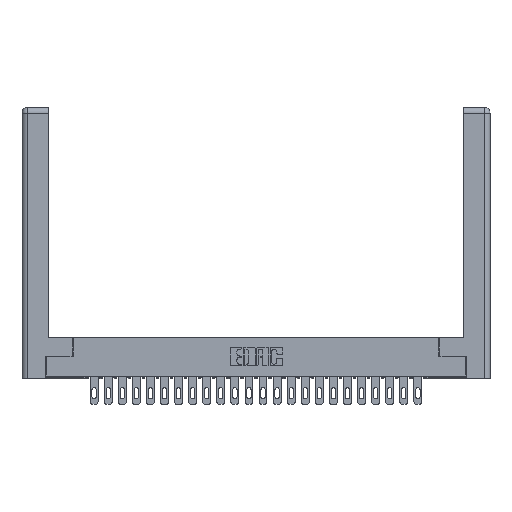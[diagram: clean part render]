
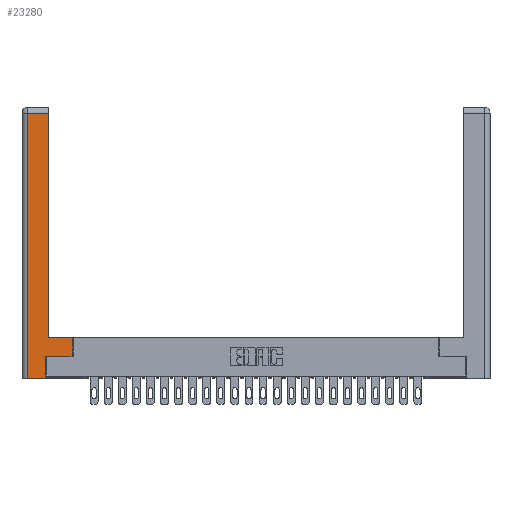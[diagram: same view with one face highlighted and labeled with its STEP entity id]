
A CAD part, top view. The second image highlights one B-rep face of the part: STEP entity #23280.
In plain terms, the highlighted planar face has unit normal (0, 0, 1).
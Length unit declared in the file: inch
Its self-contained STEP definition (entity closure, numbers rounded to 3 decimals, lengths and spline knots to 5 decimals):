
#617 = DIRECTION ( 'NONE',  ( -1., 0., 0. ) ) ;
#824 = EDGE_LOOP ( 'NONE', ( #2132, #4678, #20342, #11618, #15041, #20733, #7342, #21084 ) ) ;
#1016 = DIRECTION ( 'NONE',  ( 1., 0., 0. ) ) ;
#1511 = VECTOR ( 'NONE', #1597, 39.37008 ) ;
#1597 = DIRECTION ( 'NONE',  ( 1., 0., 0. ) ) ;
#1725 = CARTESIAN_POINT ( 'NONE',  ( 0.565, 0.245, 0. ) ) ;
#2132 = ORIENTED_EDGE ( 'NONE', *, *, #16651, .T. ) ;
#2185 = LINE ( 'NONE', #14573, #8095 ) ;
#2414 = CARTESIAN_POINT ( 'NONE',  ( 0.295, 2.94, 0. ) ) ;
#3027 = CARTESIAN_POINT ( 'NONE',  ( 0.565, 0.45, 0. ) ) ;
#3038 = DIRECTION ( 'NONE',  ( 0., 1., 0. ) ) ;
#3430 = EDGE_CURVE ( 'NONE', #23689, #16649, #26467, .T. ) ;
#3661 = CARTESIAN_POINT ( 'NONE',  ( 0.565, 0.45, 0. ) ) ;
#4438 = DIRECTION ( 'NONE',  ( -1., 0., 0. ) ) ;
#4440 = CARTESIAN_POINT ( 'NONE',  ( 0.0615, 2.94, 0. ) ) ;
#4678 = ORIENTED_EDGE ( 'NONE', *, *, #17542, .T. ) ;
#4909 = CARTESIAN_POINT ( 'NONE',  ( 0.295, 3., 0. ) ) ;
#5055 = DIRECTION ( 'NONE',  ( 0., 1., 0. ) ) ;
#5599 = DIRECTION ( 'NONE',  ( 0., 1., 0. ) ) ;
#5672 = LINE ( 'NONE', #19883, #8420 ) ;
#6234 = CARTESIAN_POINT ( 'NONE',  ( 0.265, 0.245, 0. ) ) ;
#7342 = ORIENTED_EDGE ( 'NONE', *, *, #8718, .T. ) ;
#8095 = VECTOR ( 'NONE', #8849, 39.37008 ) ;
#8358 = CARTESIAN_POINT ( 'NONE',  ( 0., 0., 0. ) ) ;
#8420 = VECTOR ( 'NONE', #3038, 39.37008 ) ;
#8718 = EDGE_CURVE ( 'NONE', #16969, #22147, #22733, .T. ) ;
#8766 = PLANE ( 'NONE',  #25941 ) ;
#8849 = DIRECTION ( 'NONE',  ( 0., -1., 0. ) ) ;
#10467 = EDGE_CURVE ( 'NONE', #22147, #15799, #21754, .T. ) ;
#11216 = LINE ( 'NONE', #4909, #23379 ) ;
#11480 = EDGE_CURVE ( 'NONE', #16649, #21962, #5672, .T. ) ;
#11585 = CARTESIAN_POINT ( 'NONE',  ( 0.295, 0.45, 0. ) ) ;
#11618 = ORIENTED_EDGE ( 'NONE', *, *, #3430, .T. ) ;
#11928 = LINE ( 'NONE', #12333, #1511 ) ;
#12333 = CARTESIAN_POINT ( 'NONE',  ( 0.565, 0.245, 0. ) ) ;
#12905 = EDGE_CURVE ( 'NONE', #21962, #16969, #11928, .T. ) ;
#13157 = CARTESIAN_POINT ( 'NONE',  ( 0.295, 0.45, 0. ) ) ;
#13964 = CARTESIAN_POINT ( 'NONE',  ( 0.265, 0., 0. ) ) ;
#14573 = CARTESIAN_POINT ( 'NONE',  ( 0.0615, 0., 0. ) ) ;
#15041 = ORIENTED_EDGE ( 'NONE', *, *, #11480, .T. ) ;
#15799 = VERTEX_POINT ( 'NONE', #11585 ) ;
#16649 = VERTEX_POINT ( 'NONE', #19810 ) ;
#16651 = EDGE_CURVE ( 'NONE', #15799, #22314, #11216, .T. ) ;
#16969 = VERTEX_POINT ( 'NONE', #1725 ) ;
#17184 = VECTOR ( 'NONE', #5599, 39.37008 ) ;
#17542 = EDGE_CURVE ( 'NONE', #22314, #25820, #23534, .T. ) ;
#17714 = VECTOR ( 'NONE', #617, 39.37008 ) ;
#18211 = VECTOR ( 'NONE', #1016, 39.37008 ) ;
#18789 = FACE_OUTER_BOUND ( 'NONE', #824, .T. ) ;
#19810 = CARTESIAN_POINT ( 'NONE',  ( 0.265, 0., 0. ) ) ;
#19883 = CARTESIAN_POINT ( 'NONE',  ( 0.265, 0.245, 0. ) ) ;
#20342 = ORIENTED_EDGE ( 'NONE', *, *, #27401, .T. ) ;
#20733 = ORIENTED_EDGE ( 'NONE', *, *, #12905, .T. ) ;
#21084 = ORIENTED_EDGE ( 'NONE', *, *, #10467, .T. ) ;
#21427 = DIRECTION ( 'NONE',  ( -1., 0., 0. ) ) ;
#21754 = LINE ( 'NONE', #13157, #17714 ) ;
#21962 = VERTEX_POINT ( 'NONE', #6234 ) ;
#22147 = VERTEX_POINT ( 'NONE', #3027 ) ;
#22314 = VERTEX_POINT ( 'NONE', #2414 ) ;
#22733 = LINE ( 'NONE', #3661, #17184 ) ;
#23280 = ADVANCED_FACE ( 'NONE', ( #18789 ), #8766, .F. ) ;
#23379 = VECTOR ( 'NONE', #5055, 39.37008 ) ;
#23534 = LINE ( 'NONE', #4440, #24297 ) ;
#23689 = VERTEX_POINT ( 'NONE', #25450 ) ;
#24297 = VECTOR ( 'NONE', #21427, 39.37008 ) ;
#24401 = CARTESIAN_POINT ( 'NONE',  ( 0.0615, 2.94, 0. ) ) ;
#25450 = CARTESIAN_POINT ( 'NONE',  ( 0.0615, 0., 0. ) ) ;
#25615 = DIRECTION ( 'NONE',  ( 0., 0., -1. ) ) ;
#25820 = VERTEX_POINT ( 'NONE', #24401 ) ;
#25941 = AXIS2_PLACEMENT_3D ( 'NONE', #8358, #25615, #4438 ) ;
#26467 = LINE ( 'NONE', #13964, #18211 ) ;
#27401 = EDGE_CURVE ( 'NONE', #25820, #23689, #2185, .T. ) ;
